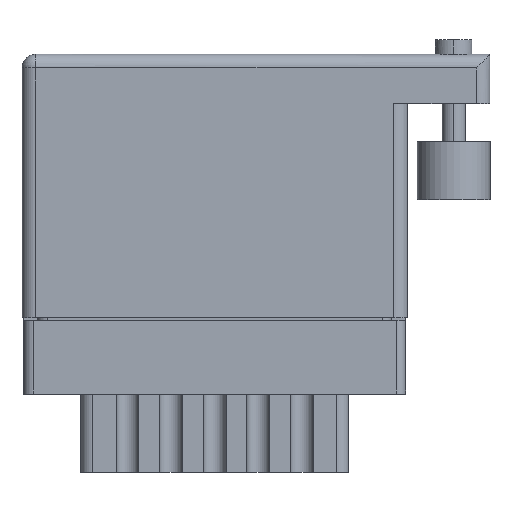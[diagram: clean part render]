
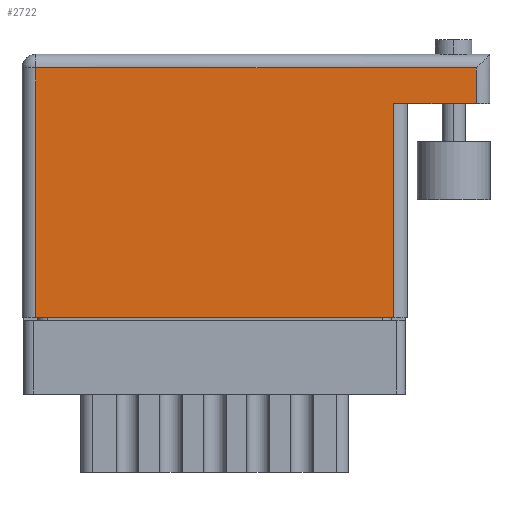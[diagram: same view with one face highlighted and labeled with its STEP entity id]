
A CAD part, front view. The second image highlights one B-rep face of the part: STEP entity #2722.
In plain terms, the highlighted face is planar.
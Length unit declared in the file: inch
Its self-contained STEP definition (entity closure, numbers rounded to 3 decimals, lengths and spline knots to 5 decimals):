
#235 = VECTOR ( 'NONE', #17835, 39.37008 ) ;
#953 = EDGE_CURVE ( 'NONE', #22865, #17248, #15589, .T. ) ;
#2122 = FACE_OUTER_BOUND ( 'NONE', #15425, .T. ) ;
#2488 = CARTESIAN_POINT ( 'NONE',  ( 1.278, 0., 0. ) ) ;
#2722 = ADVANCED_FACE ( 'NONE', ( #2122 ), #16953, .F. ) ;
#3239 = EDGE_CURVE ( 'NONE', #19142, #16459, #23247, .T. ) ;
#3300 = EDGE_CURVE ( 'NONE', #17248, #18294, #9082, .T. ) ;
#3389 = VECTOR ( 'NONE', #24390, 39.37008 ) ;
#4059 = CARTESIAN_POINT ( 'NONE',  ( 0.047, 0., 0. ) ) ;
#4113 = DIRECTION ( 'NONE',  ( 0., 1., 0. ) ) ;
#4531 = ORIENTED_EDGE ( 'NONE', *, *, #953, .T. ) ;
#5133 = ORIENTED_EDGE ( 'NONE', *, *, #3239, .F. ) ;
#5232 = CARTESIAN_POINT ( 'NONE',  ( 1.562, 0.859, 0. ) ) ;
#5914 = VECTOR ( 'NONE', #16921, 39.37008 ) ;
#6813 = CARTESIAN_POINT ( 'NONE',  ( 1.609, 0.736, 0. ) ) ;
#7013 = CARTESIAN_POINT ( 'NONE',  ( 0., 0.906, 0. ) ) ;
#7293 = CARTESIAN_POINT ( 'NONE',  ( 1.562, 0.736, 0. ) ) ;
#9082 = LINE ( 'NONE', #23108, #25121 ) ;
#9388 = LINE ( 'NONE', #10031, #235 ) ;
#10022 = CARTESIAN_POINT ( 'NONE',  ( 1.562, 0.906, 0. ) ) ;
#10031 = CARTESIAN_POINT ( 'NONE',  ( 1.278, 0.736, 0. ) ) ;
#10216 = AXIS2_PLACEMENT_3D ( 'NONE', #7013, #17288, #21155 ) ;
#10971 = VERTEX_POINT ( 'NONE', #5232 ) ;
#11578 = ORIENTED_EDGE ( 'NONE', *, *, #3300, .T. ) ;
#12561 = CARTESIAN_POINT ( 'NONE',  ( 0., 0.859, 0. ) ) ;
#15425 = EDGE_LOOP ( 'NONE', ( #11578, #25784, #5133, #19987, #25253, #4531 ) ) ;
#15589 = LINE ( 'NONE', #4059, #17460 ) ;
#15805 = LINE ( 'NONE', #10022, #24944 ) ;
#16459 = VERTEX_POINT ( 'NONE', #25960 ) ;
#16921 = DIRECTION ( 'NONE',  ( -1., 0., 0. ) ) ;
#16953 = PLANE ( 'NONE',  #10216 ) ;
#17248 = VERTEX_POINT ( 'NONE', #23165 ) ;
#17288 = DIRECTION ( 'NONE',  ( 0., 0., -1. ) ) ;
#17460 = VECTOR ( 'NONE', #22267, 39.37008 ) ;
#17835 = DIRECTION ( 'NONE',  ( 0., 1., 0. ) ) ;
#17870 = LINE ( 'NONE', #12561, #3389 ) ;
#18294 = VERTEX_POINT ( 'NONE', #2488 ) ;
#19142 = VERTEX_POINT ( 'NONE', #7293 ) ;
#19987 = ORIENTED_EDGE ( 'NONE', *, *, #23510, .T. ) ;
#20264 = CARTESIAN_POINT ( 'NONE',  ( 0.047, 0.859, 0. ) ) ;
#21126 = DIRECTION ( 'NONE',  ( 1., 0., 0. ) ) ;
#21155 = DIRECTION ( 'NONE',  ( -1., 0., 0. ) ) ;
#22267 = DIRECTION ( 'NONE',  ( 0., -1., 0. ) ) ;
#22865 = VERTEX_POINT ( 'NONE', #20264 ) ;
#23108 = CARTESIAN_POINT ( 'NONE',  ( 0., 0., 0. ) ) ;
#23165 = CARTESIAN_POINT ( 'NONE',  ( 0.047, 0., 0. ) ) ;
#23247 = LINE ( 'NONE', #6813, #5914 ) ;
#23510 = EDGE_CURVE ( 'NONE', #19142, #10971, #15805, .T. ) ;
#24390 = DIRECTION ( 'NONE',  ( -1., 0., 0. ) ) ;
#24944 = VECTOR ( 'NONE', #4113, 39.37008 ) ;
#25094 = EDGE_CURVE ( 'NONE', #18294, #16459, #9388, .T. ) ;
#25121 = VECTOR ( 'NONE', #21126, 39.37008 ) ;
#25180 = EDGE_CURVE ( 'NONE', #10971, #22865, #17870, .T. ) ;
#25253 = ORIENTED_EDGE ( 'NONE', *, *, #25180, .T. ) ;
#25784 = ORIENTED_EDGE ( 'NONE', *, *, #25094, .T. ) ;
#25960 = CARTESIAN_POINT ( 'NONE',  ( 1.278, 0.736, 0. ) ) ;
